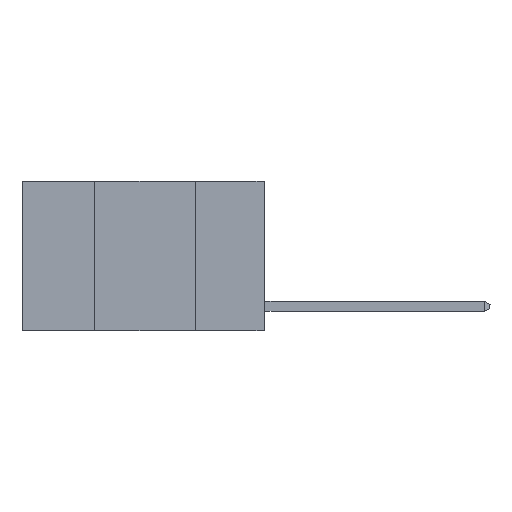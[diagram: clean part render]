
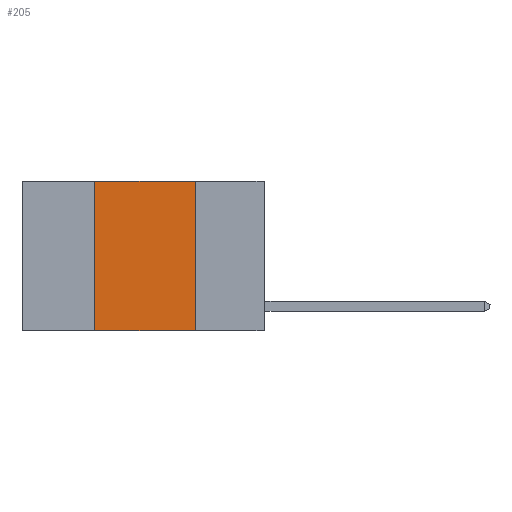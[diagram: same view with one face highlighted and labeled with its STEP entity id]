
A CAD part, left-side view. The second image highlights one B-rep face of the part: STEP entity #205.
In plain terms, the highlighted planar face has unit normal (-1, 0, 0).
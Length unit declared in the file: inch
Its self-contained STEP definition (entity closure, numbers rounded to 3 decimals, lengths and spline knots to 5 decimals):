
#205 = ADVANCED_FACE ( 'NONE', ( #13843 ), #7646, .F. ) ;
#1776 = VECTOR ( 'NONE', #2266, 39.37008 ) ;
#2266 = DIRECTION ( 'NONE',  ( 0., -1., 0. ) ) ;
#2794 = ORIENTED_EDGE ( 'NONE', *, *, #11764, .T. ) ;
#2821 = DIRECTION ( 'NONE',  ( 0., 0., 1. ) ) ;
#3236 = VECTOR ( 'NONE', #7389, 39.37008 ) ;
#3853 = CARTESIAN_POINT ( 'NONE',  ( 0., 0.6, 0. ) ) ;
#4220 = EDGE_CURVE ( 'NONE', #14069, #15139, #13880, .T. ) ;
#4489 = ORIENTED_EDGE ( 'NONE', *, *, #13164, .F. ) ;
#5418 = CARTESIAN_POINT ( 'NONE',  ( 0., 0.42, 0. ) ) ;
#5915 = ORIENTED_EDGE ( 'NONE', *, *, #12463, .F. ) ;
#5953 = VECTOR ( 'NONE', #2821, 39.37008 ) ;
#6673 = ORIENTED_EDGE ( 'NONE', *, *, #4220, .F. ) ;
#6954 = DIRECTION ( 'NONE',  ( 0., -1., 0. ) ) ;
#7389 = DIRECTION ( 'NONE',  ( 0., 0., -1. ) ) ;
#7646 = PLANE ( 'NONE',  #8776 ) ;
#8733 = CARTESIAN_POINT ( 'NONE',  ( 0., 0.6, -0.37 ) ) ;
#8776 = AXIS2_PLACEMENT_3D ( 'NONE', #3853, #11507, #13071 ) ;
#9723 = VECTOR ( 'NONE', #6954, 39.37008 ) ;
#10765 = LINE ( 'NONE', #14799, #9723 ) ;
#11507 = DIRECTION ( 'NONE',  ( 1., 0., 0. ) ) ;
#11687 = CARTESIAN_POINT ( 'NONE',  ( 0., 0.17, 0. ) ) ;
#11764 = EDGE_CURVE ( 'NONE', #13624, #15139, #12444, .T. ) ;
#12016 = EDGE_LOOP ( 'NONE', ( #6673, #4489, #5915, #2794 ) ) ;
#12116 = CARTESIAN_POINT ( 'NONE',  ( 0., 0.42, -0.37 ) ) ;
#12444 = LINE ( 'NONE', #8733, #1776 ) ;
#12463 = EDGE_CURVE ( 'NONE', #13624, #14721, #12746, .T. ) ;
#12746 = LINE ( 'NONE', #5418, #5953 ) ;
#13071 = DIRECTION ( 'NONE',  ( 0., 0., -1. ) ) ;
#13164 = EDGE_CURVE ( 'NONE', #14721, #14069, #10765, .T. ) ;
#13226 = CARTESIAN_POINT ( 'NONE',  ( 0., 0.17, 0. ) ) ;
#13624 = VERTEX_POINT ( 'NONE', #12116 ) ;
#13843 = FACE_OUTER_BOUND ( 'NONE', #12016, .T. ) ;
#13880 = LINE ( 'NONE', #13226, #3236 ) ;
#14069 = VERTEX_POINT ( 'NONE', #11687 ) ;
#14604 = CARTESIAN_POINT ( 'NONE',  ( 0., 0.17, -0.37 ) ) ;
#14721 = VERTEX_POINT ( 'NONE', #14728 ) ;
#14728 = CARTESIAN_POINT ( 'NONE',  ( 0., 0.42, 0. ) ) ;
#14799 = CARTESIAN_POINT ( 'NONE',  ( 0., 0.6, 0. ) ) ;
#15139 = VERTEX_POINT ( 'NONE', #14604 ) ;
